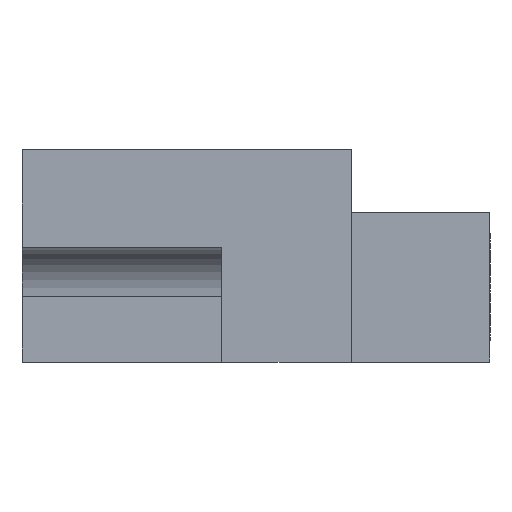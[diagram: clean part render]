
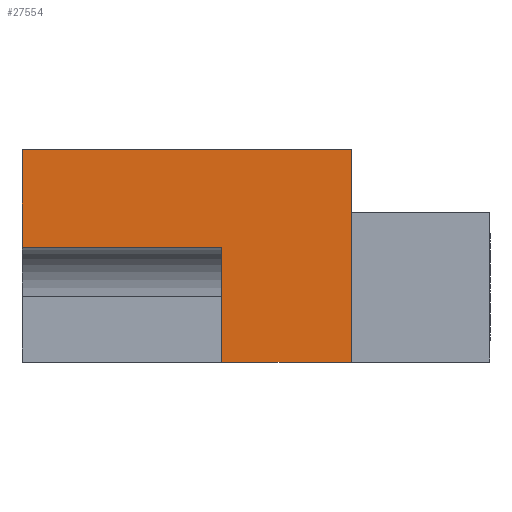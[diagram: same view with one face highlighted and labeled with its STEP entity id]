
A CAD part, left-side view. The second image highlights one B-rep face of the part: STEP entity #27554.
In plain terms, the highlighted planar face has unit normal (-1, 0, 0).
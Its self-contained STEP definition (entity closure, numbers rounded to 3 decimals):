
#1412 = VECTOR ( 'NONE', #35213, 1000. ) ;
#1455 = DIRECTION ( 'NONE',  ( 0., 0., -1. ) ) ;
#2640 = ORIENTED_EDGE ( 'NONE', *, *, #3642, .F. ) ;
#3031 = VECTOR ( 'NONE', #14406, 1000. ) ;
#3360 = EDGE_CURVE ( 'NONE', #10487, #31418, #9539, .T. ) ;
#3642 = EDGE_CURVE ( 'NONE', #36190, #40854, #21302, .T. ) ;
#3901 = CARTESIAN_POINT ( 'NONE',  ( 0., 0., -13.487 ) ) ;
#7798 = EDGE_CURVE ( 'NONE', #31418, #36190, #25723, .T. ) ;
#8255 = AXIS2_PLACEMENT_3D ( 'NONE', #16130, #39000, #19434 ) ;
#9539 = LINE ( 'NONE', #38635, #1412 ) ;
#10487 = VERTEX_POINT ( 'NONE', #34134 ) ;
#12170 = VECTOR ( 'NONE', #22866, 1000. ) ;
#13316 = CARTESIAN_POINT ( 'NONE',  ( 0., 8.255, -13.487 ) ) ;
#13826 = EDGE_CURVE ( 'NONE', #19742, #10487, #24980, .T. ) ;
#14267 = ORIENTED_EDGE ( 'NONE', *, *, #37192, .F. ) ;
#14406 = DIRECTION ( 'NONE',  ( 0., 1., 0. ) ) ;
#15142 = VECTOR ( 'NONE', #35087, 1000. ) ;
#16130 = CARTESIAN_POINT ( 'NONE',  ( 0., 0., 0. ) ) ;
#16860 = FACE_OUTER_BOUND ( 'NONE', #28269, .T. ) ;
#17872 = ORIENTED_EDGE ( 'NONE', *, *, #7798, .F. ) ;
#18746 = ORIENTED_EDGE ( 'NONE', *, *, #13826, .F. ) ;
#19434 = DIRECTION ( 'NONE',  ( 0., 0., -1. ) ) ;
#19742 = VERTEX_POINT ( 'NONE', #25568 ) ;
#20860 = LINE ( 'NONE', #13316, #39264 ) ;
#21302 = LINE ( 'NONE', #25220, #15142 ) ;
#22688 = CARTESIAN_POINT ( 'NONE',  ( 0., 8.255, -13.487 ) ) ;
#22866 = DIRECTION ( 'NONE',  ( 0., 0., 1. ) ) ;
#24306 = CARTESIAN_POINT ( 'NONE',  ( 0., 0., 0. ) ) ;
#24980 = LINE ( 'NONE', #29870, #12170 ) ;
#25160 = EDGE_CURVE ( 'NONE', #40291, #19742, #25541, .T. ) ;
#25220 = CARTESIAN_POINT ( 'NONE',  ( 0., -8.814, -13.487 ) ) ;
#25541 = LINE ( 'NONE', #34453, #3031 ) ;
#25568 = CARTESIAN_POINT ( 'NONE',  ( 0., 20.955, -6.172 ) ) ;
#25723 = LINE ( 'NONE', #24306, #31918 ) ;
#27554 = ADVANCED_FACE ( 'NONE', ( #16860 ), #39288, .F. ) ;
#28269 = EDGE_LOOP ( 'NONE', ( #2640, #17872, #37835, #18746, #33107, #14267 ) ) ;
#29199 = CARTESIAN_POINT ( 'NONE',  ( 0., 0., 0. ) ) ;
#29870 = CARTESIAN_POINT ( 'NONE',  ( 0., 20.955, -13.487 ) ) ;
#31418 = VERTEX_POINT ( 'NONE', #29199 ) ;
#31918 = VECTOR ( 'NONE', #1455, 1000. ) ;
#33107 = ORIENTED_EDGE ( 'NONE', *, *, #25160, .F. ) ;
#34134 = CARTESIAN_POINT ( 'NONE',  ( 0., 20.955, 0. ) ) ;
#34453 = CARTESIAN_POINT ( 'NONE',  ( 0., 8.255, -6.172 ) ) ;
#35087 = DIRECTION ( 'NONE',  ( 0., 1., 0. ) ) ;
#35213 = DIRECTION ( 'NONE',  ( 0., -1., 0. ) ) ;
#35330 = CARTESIAN_POINT ( 'NONE',  ( 0., 8.255, -6.172 ) ) ;
#36190 = VERTEX_POINT ( 'NONE', #3901 ) ;
#36380 = DIRECTION ( 'NONE',  ( 0., 0., 1. ) ) ;
#37192 = EDGE_CURVE ( 'NONE', #40854, #40291, #20860, .T. ) ;
#37835 = ORIENTED_EDGE ( 'NONE', *, *, #3360, .F. ) ;
#38635 = CARTESIAN_POINT ( 'NONE',  ( 0., 11.506, 0. ) ) ;
#39000 = DIRECTION ( 'NONE',  ( 1., 0., 0. ) ) ;
#39264 = VECTOR ( 'NONE', #36380, 1000. ) ;
#39288 = PLANE ( 'NONE',  #8255 ) ;
#40291 = VERTEX_POINT ( 'NONE', #35330 ) ;
#40854 = VERTEX_POINT ( 'NONE', #22688 ) ;
